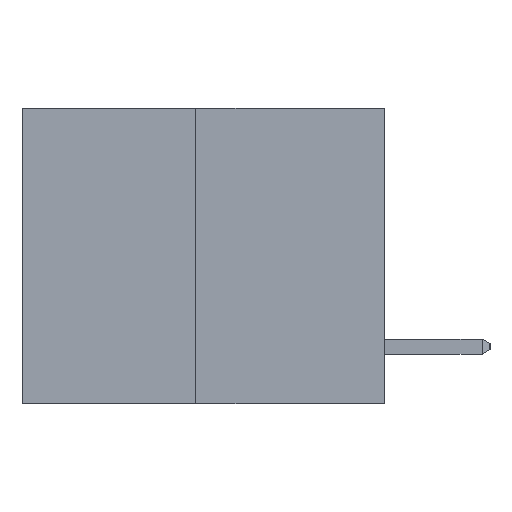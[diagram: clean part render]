
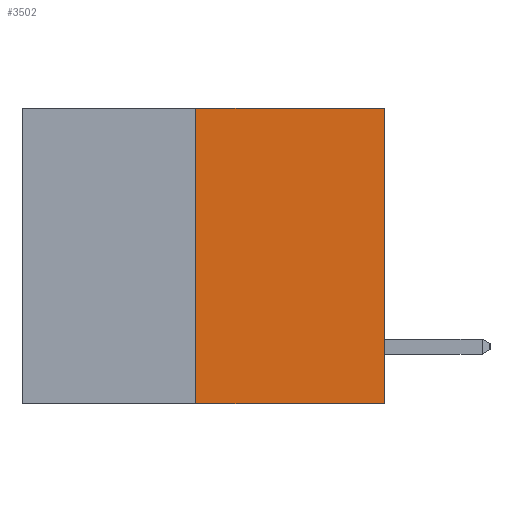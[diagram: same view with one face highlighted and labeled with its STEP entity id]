
A CAD part, left-side view. The second image highlights one B-rep face of the part: STEP entity #3502.
In plain terms, the highlighted planar face has unit normal (-1, 0, 0).
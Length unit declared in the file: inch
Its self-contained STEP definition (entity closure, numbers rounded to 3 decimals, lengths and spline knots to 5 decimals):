
#62 = DIRECTION ( 'NONE',  ( 0., 0., 1. ) ) ;
#234 = ORIENTED_EDGE ( 'NONE', *, *, #10191, .F. ) ;
#270 = LINE ( 'NONE', #8338, #4077 ) ;
#524 = CARTESIAN_POINT ( 'NONE',  ( 0., 0.6, -0.49 ) ) ;
#759 = CARTESIAN_POINT ( 'NONE',  ( 0., 0., 0. ) ) ;
#961 = DIRECTION ( 'NONE',  ( 1., 0., 0. ) ) ;
#1026 = DIRECTION ( 'NONE',  ( 0., 0., -1. ) ) ;
#1125 = LINE ( 'NONE', #759, #9492 ) ;
#1126 = AXIS2_PLACEMENT_3D ( 'NONE', #2664, #961, #1026 ) ;
#1442 = CARTESIAN_POINT ( 'NONE',  ( 0., 0.312, 0. ) ) ;
#2067 = DIRECTION ( 'NONE',  ( 0., -1., 0. ) ) ;
#2396 = VERTEX_POINT ( 'NONE', #9186 ) ;
#2442 = EDGE_CURVE ( 'NONE', #9724, #9336, #3448, .T. ) ;
#2454 = EDGE_LOOP ( 'NONE', ( #234, #8351, #3486, #5544 ) ) ;
#2664 = CARTESIAN_POINT ( 'NONE',  ( 0., 0.6, 0. ) ) ;
#3199 = EDGE_CURVE ( 'NONE', #3569, #9336, #1125, .T. ) ;
#3448 = LINE ( 'NONE', #8508, #5585 ) ;
#3486 = ORIENTED_EDGE ( 'NONE', *, *, #3199, .T. ) ;
#3502 = ADVANCED_FACE ( 'NONE', ( #10494 ), #6678, .F. ) ;
#3569 = VERTEX_POINT ( 'NONE', #10064 ) ;
#3897 = LINE ( 'NONE', #524, #6836 ) ;
#4077 = VECTOR ( 'NONE', #62, 39.37008 ) ;
#5496 = DIRECTION ( 'NONE',  ( 0., -1., 0. ) ) ;
#5544 = ORIENTED_EDGE ( 'NONE', *, *, #2442, .F. ) ;
#5585 = VECTOR ( 'NONE', #2067, 39.37008 ) ;
#6243 = EDGE_CURVE ( 'NONE', #2396, #3569, #3897, .T. ) ;
#6678 = PLANE ( 'NONE',  #1126 ) ;
#6836 = VECTOR ( 'NONE', #5496, 39.37008 ) ;
#8169 = DIRECTION ( 'NONE',  ( 0., 0., 1. ) ) ;
#8338 = CARTESIAN_POINT ( 'NONE',  ( 0., 0.312, -0.49 ) ) ;
#8351 = ORIENTED_EDGE ( 'NONE', *, *, #6243, .T. ) ;
#8508 = CARTESIAN_POINT ( 'NONE',  ( 0., 0.6, 0. ) ) ;
#9186 = CARTESIAN_POINT ( 'NONE',  ( 0., 0.312, -0.49 ) ) ;
#9336 = VERTEX_POINT ( 'NONE', #9523 ) ;
#9492 = VECTOR ( 'NONE', #8169, 39.37008 ) ;
#9523 = CARTESIAN_POINT ( 'NONE',  ( 0., 0., 0. ) ) ;
#9724 = VERTEX_POINT ( 'NONE', #1442 ) ;
#10064 = CARTESIAN_POINT ( 'NONE',  ( 0., 0., -0.49 ) ) ;
#10191 = EDGE_CURVE ( 'NONE', #2396, #9724, #270, .T. ) ;
#10494 = FACE_OUTER_BOUND ( 'NONE', #2454, .T. ) ;
